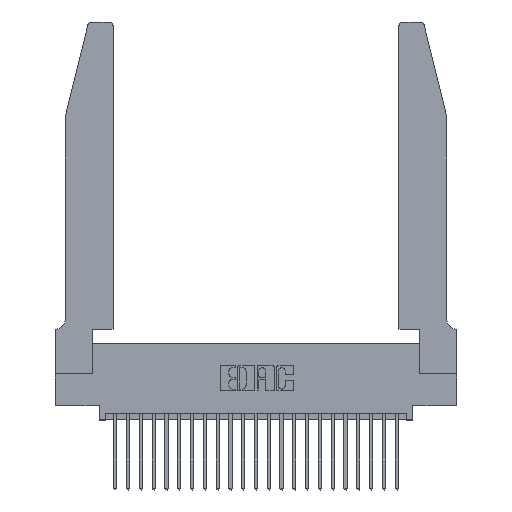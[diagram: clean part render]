
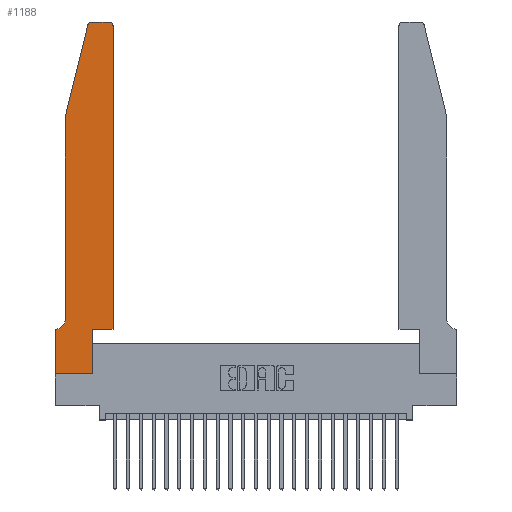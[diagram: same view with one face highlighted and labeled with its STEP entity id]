
A CAD part, top view. The second image highlights one B-rep face of the part: STEP entity #1188.
In plain terms, the highlighted planar face has unit normal (0, 0, 1).
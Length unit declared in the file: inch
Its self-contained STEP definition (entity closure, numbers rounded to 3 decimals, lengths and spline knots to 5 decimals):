
#616 = DIRECTION ( 'NONE',  ( 1., 0., 0. ) ) ;
#829 = CARTESIAN_POINT ( 'NONE',  ( 0.4205, 2.72, 0.37 ) ) ;
#982 = CARTESIAN_POINT ( 'NONE',  ( 0.2605, 2.75, 0.37 ) ) ;
#1188 = ADVANCED_FACE ( 'NONE', ( #7075 ), #4210, .T. ) ;
#1396 = VERTEX_POINT ( 'NONE', #3905 ) ;
#1591 = CIRCLE ( 'NONE', #5634, 0.03 ) ;
#2202 = CARTESIAN_POINT ( 'NONE',  ( 0.4205, 2.75, 0.37 ) ) ;
#2844 = DIRECTION ( 'NONE',  ( 1., 0., 0. ) ) ;
#2881 = VECTOR ( 'NONE', #20080, 39.37008 ) ;
#2883 = DIRECTION ( 'NONE',  ( 0., 0., 1. ) ) ;
#2937 = ORIENTED_EDGE ( 'NONE', *, *, #14453, .T. ) ;
#3324 = LINE ( 'NONE', #9387, #18509 ) ;
#3414 = EDGE_CURVE ( 'NONE', #25452, #1396, #11681, .T. ) ;
#3905 = CARTESIAN_POINT ( 'NONE',  ( 0.0755, 0.42, 0.37 ) ) ;
#3979 = VERTEX_POINT ( 'NONE', #19639 ) ;
#4012 = CIRCLE ( 'NONE', #12813, 0.03 ) ;
#4043 = LINE ( 'NONE', #17597, #19871 ) ;
#4210 = PLANE ( 'NONE',  #8194 ) ;
#4588 = DIRECTION ( 'NONE',  ( 0., 1., 0. ) ) ;
#4604 = VERTEX_POINT ( 'NONE', #19866 ) ;
#4764 = CARTESIAN_POINT ( 'NONE',  ( 0.2865, 0., 0.37 ) ) ;
#4790 = VERTEX_POINT ( 'NONE', #4764 ) ;
#5186 = DIRECTION ( 'NONE',  ( 0., 0., -1. ) ) ;
#5481 = ORIENTED_EDGE ( 'NONE', *, *, #10785, .T. ) ;
#5634 = AXIS2_PLACEMENT_3D ( 'NONE', #14723, #2883, #16737 ) ;
#5724 = VERTEX_POINT ( 'NONE', #7654 ) ;
#6082 = VERTEX_POINT ( 'NONE', #6675 ) ;
#6421 = VECTOR ( 'NONE', #13647, 39.37008 ) ;
#6453 = VERTEX_POINT ( 'NONE', #2202 ) ;
#6675 = CARTESIAN_POINT ( 'NONE',  ( 0., 0.35, 0.37 ) ) ;
#6736 = LINE ( 'NONE', #23719, #16066 ) ;
#6780 = VECTOR ( 'NONE', #616, 39.37008 ) ;
#7075 = FACE_OUTER_BOUND ( 'NONE', #17135, .T. ) ;
#7178 = DIRECTION ( 'NONE',  ( 1., 0., 0. ) ) ;
#7654 = CARTESIAN_POINT ( 'NONE',  ( 0.4505, 2.72, 0.37 ) ) ;
#7694 = DIRECTION ( 'NONE',  ( 0., 0., 1. ) ) ;
#8044 = VECTOR ( 'NONE', #4588, 39.37008 ) ;
#8194 = AXIS2_PLACEMENT_3D ( 'NONE', #10239, #7694, #7178 ) ;
#8260 = AXIS2_PLACEMENT_3D ( 'NONE', #17063, #5186, #19081 ) ;
#8927 = LINE ( 'NONE', #12759, #18274 ) ;
#9133 = ORIENTED_EDGE ( 'NONE', *, *, #16009, .T. ) ;
#9387 = CARTESIAN_POINT ( 'NONE',  ( 0.0755, 2., 0.37 ) ) ;
#9919 = ORIENTED_EDGE ( 'NONE', *, *, #22061, .T. ) ;
#9963 = VERTEX_POINT ( 'NONE', #15886 ) ;
#10239 = CARTESIAN_POINT ( 'NONE',  ( 0., 0.35, 0.37 ) ) ;
#10487 = VERTEX_POINT ( 'NONE', #19355 ) ;
#10785 = EDGE_CURVE ( 'NONE', #9963, #4790, #13397, .T. ) ;
#11333 = ORIENTED_EDGE ( 'NONE', *, *, #16618, .T. ) ;
#11681 = LINE ( 'NONE', #23479, #6421 ) ;
#11924 = VECTOR ( 'NONE', #18853, 39.37008 ) ;
#12156 = EDGE_CURVE ( 'NONE', #21312, #5724, #12682, .T. ) ;
#12226 = CARTESIAN_POINT ( 'NONE',  ( 0.0055, 0.35, 0.37 ) ) ;
#12427 = CARTESIAN_POINT ( 'NONE',  ( 0.4505, 0.35, 0.37 ) ) ;
#12505 = ORIENTED_EDGE ( 'NONE', *, *, #21749, .T. ) ;
#12682 = LINE ( 'NONE', #12427, #8044 ) ;
#12759 = CARTESIAN_POINT ( 'NONE',  ( 0., 0., 0.37 ) ) ;
#12813 = AXIS2_PLACEMENT_3D ( 'NONE', #829, #14682, #2844 ) ;
#12818 = EDGE_CURVE ( 'NONE', #6082, #9963, #8927, .T. ) ;
#13397 = LINE ( 'NONE', #14078, #2881 ) ;
#13577 = DIRECTION ( 'NONE',  ( 0., 1., 0. ) ) ;
#13629 = ORIENTED_EDGE ( 'NONE', *, *, #12818, .T. ) ;
#13647 = DIRECTION ( 'NONE',  ( 0., -1., 0. ) ) ;
#13891 = DIRECTION ( 'NONE',  ( -1., 0., 0. ) ) ;
#14078 = CARTESIAN_POINT ( 'NONE',  ( 0., 0., 0.37 ) ) ;
#14453 = EDGE_CURVE ( 'NONE', #4604, #25452, #3324, .T. ) ;
#14526 = ORIENTED_EDGE ( 'NONE', *, *, #23010, .T. ) ;
#14682 = DIRECTION ( 'NONE',  ( 0., 0., 1. ) ) ;
#14723 = CARTESIAN_POINT ( 'NONE',  ( 0.284, 2.72, 0.37 ) ) ;
#14771 = DIRECTION ( 'NONE',  ( 0., -1., 0. ) ) ;
#15117 = ORIENTED_EDGE ( 'NONE', *, *, #21928, .T. ) ;
#15886 = CARTESIAN_POINT ( 'NONE',  ( 0., 0., 0.37 ) ) ;
#16009 = EDGE_CURVE ( 'NONE', #5724, #6453, #4012, .T. ) ;
#16066 = VECTOR ( 'NONE', #13891, 39.37008 ) ;
#16618 = EDGE_CURVE ( 'NONE', #20940, #6082, #6736, .T. ) ;
#16737 = DIRECTION ( 'NONE',  ( 1., 0., 0. ) ) ;
#17063 = CARTESIAN_POINT ( 'NONE',  ( 0.0055, 0.42, 0.37 ) ) ;
#17100 = ORIENTED_EDGE ( 'NONE', *, *, #12156, .T. ) ;
#17135 = EDGE_LOOP ( 'NONE', ( #17143, #12505, #2937, #20068, #15117, #11333, #13629, #5481, #9919, #14526, #17100, #9133 ) ) ;
#17143 = ORIENTED_EDGE ( 'NONE', *, *, #25312, .T. ) ;
#17246 = LINE ( 'NONE', #982, #11924 ) ;
#17384 = CARTESIAN_POINT ( 'NONE',  ( 0.4505, 0.35, 0.37 ) ) ;
#17408 = DIRECTION ( 'NONE',  ( -0.239, -0.971, 0. ) ) ;
#17597 = CARTESIAN_POINT ( 'NONE',  ( 0.2865, 0.35, 0.37 ) ) ;
#18274 = VECTOR ( 'NONE', #14771, 39.37008 ) ;
#18315 = CIRCLE ( 'NONE', #8260, 0.07 ) ;
#18509 = VECTOR ( 'NONE', #17408, 39.37008 ) ;
#18614 = LINE ( 'NONE', #24272, #6780 ) ;
#18853 = DIRECTION ( 'NONE',  ( -1., 0., 0. ) ) ;
#19081 = DIRECTION ( 'NONE',  ( -1., 0., 0. ) ) ;
#19355 = CARTESIAN_POINT ( 'NONE',  ( 0.2865, 0.35, 0.37 ) ) ;
#19639 = CARTESIAN_POINT ( 'NONE',  ( 0.284, 2.75, 0.37 ) ) ;
#19866 = CARTESIAN_POINT ( 'NONE',  ( 0.25487, 2.72718, 0.37 ) ) ;
#19871 = VECTOR ( 'NONE', #13577, 39.37008 ) ;
#20068 = ORIENTED_EDGE ( 'NONE', *, *, #3414, .T. ) ;
#20080 = DIRECTION ( 'NONE',  ( 1., 0., 0. ) ) ;
#20940 = VERTEX_POINT ( 'NONE', #12226 ) ;
#21157 = CARTESIAN_POINT ( 'NONE',  ( 0.0755, 2., 0.37 ) ) ;
#21312 = VERTEX_POINT ( 'NONE', #17384 ) ;
#21749 = EDGE_CURVE ( 'NONE', #3979, #4604, #1591, .T. ) ;
#21928 = EDGE_CURVE ( 'NONE', #1396, #20940, #18315, .T. ) ;
#22061 = EDGE_CURVE ( 'NONE', #4790, #10487, #4043, .T. ) ;
#23010 = EDGE_CURVE ( 'NONE', #10487, #21312, #18614, .T. ) ;
#23479 = CARTESIAN_POINT ( 'NONE',  ( 0.0755, 2., 0.37 ) ) ;
#23719 = CARTESIAN_POINT ( 'NONE',  ( 0.0755, 0.35, 0.37 ) ) ;
#24272 = CARTESIAN_POINT ( 'NONE',  ( 0.4505, 0.35, 0.37 ) ) ;
#25312 = EDGE_CURVE ( 'NONE', #6453, #3979, #17246, .T. ) ;
#25452 = VERTEX_POINT ( 'NONE', #21157 ) ;
